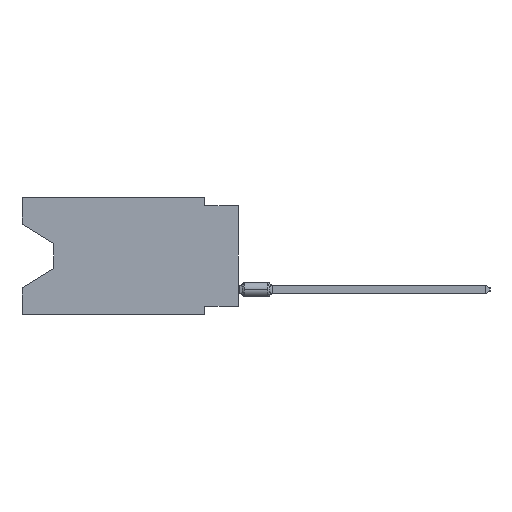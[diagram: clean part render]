
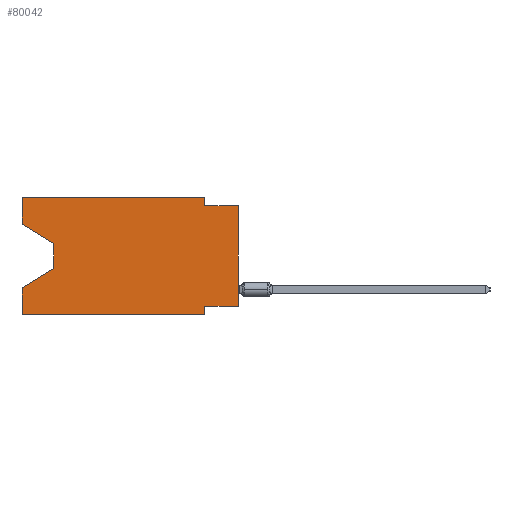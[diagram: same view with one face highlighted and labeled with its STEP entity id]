
A CAD part, left-side view. The second image highlights one B-rep face of the part: STEP entity #80042.
In plain terms, the highlighted planar face has unit normal (-1, 0, 0).
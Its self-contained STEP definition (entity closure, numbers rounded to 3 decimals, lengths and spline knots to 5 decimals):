
#1138 = CARTESIAN_POINT ( 'NONE',  ( 0., 0.645, 0. ) ) ;
#2386 = DIRECTION ( 'NONE',  ( 0., 0., -1. ) ) ;
#5109 = EDGE_CURVE ( 'NONE', #22256, #36637, #84031, .T. ) ;
#5518 = CARTESIAN_POINT ( 'NONE',  ( 0., 0.1, -0.35 ) ) ;
#6136 = VECTOR ( 'NONE', #38522, 39.37008 ) ;
#7480 = PLANE ( 'NONE',  #61533 ) ;
#9492 = VECTOR ( 'NONE', #92380, 39.37008 ) ;
#10822 = VERTEX_POINT ( 'NONE', #35926 ) ;
#14160 = CARTESIAN_POINT ( 'NONE',  ( 0., 0.645, 0. ) ) ;
#16501 = DIRECTION ( 'NONE',  ( 0., 0., 1. ) ) ;
#17333 = ORIENTED_EDGE ( 'NONE', *, *, #82261, .F. ) ;
#17602 = VECTOR ( 'NONE', #30311, 39.37008 ) ;
#21684 = ORIENTED_EDGE ( 'NONE', *, *, #89565, .F. ) ;
#22223 = CARTESIAN_POINT ( 'NONE',  ( 0., 0., -0.025 ) ) ;
#22256 = VERTEX_POINT ( 'NONE', #79996 ) ;
#23009 = DIRECTION ( 'NONE',  ( 0., -0.855, -0.519 ) ) ;
#23027 = EDGE_CURVE ( 'NONE', #95445, #22256, #58249, .T. ) ;
#23307 = DIRECTION ( 'NONE',  ( 1., 0., 0. ) ) ;
#24504 = ORIENTED_EDGE ( 'NONE', *, *, #60805, .T. ) ;
#24520 = CARTESIAN_POINT ( 'NONE',  ( 0., 0.645, -0.08025 ) ) ;
#25581 = LINE ( 'NONE', #94180, #74170 ) ;
#26067 = CARTESIAN_POINT ( 'NONE',  ( 0., 0.645, -0.26975 ) ) ;
#27872 = ORIENTED_EDGE ( 'NONE', *, *, #70523, .F. ) ;
#28115 = VERTEX_POINT ( 'NONE', #47231 ) ;
#30311 = DIRECTION ( 'NONE',  ( 0., 0., -1. ) ) ;
#30899 = EDGE_CURVE ( 'NONE', #37259, #60543, #55387, .T. ) ;
#31280 = DIRECTION ( 'NONE',  ( 0., 0.855, -0.519 ) ) ;
#31504 = EDGE_CURVE ( 'NONE', #95445, #28115, #61188, .T. ) ;
#31776 = LINE ( 'NONE', #55344, #57600 ) ;
#35926 = CARTESIAN_POINT ( 'NONE',  ( 0., 0.55, -0.212 ) ) ;
#36637 = VERTEX_POINT ( 'NONE', #5518 ) ;
#37259 = VERTEX_POINT ( 'NONE', #79303 ) ;
#38190 = FACE_OUTER_BOUND ( 'NONE', #45437, .T. ) ;
#38522 = DIRECTION ( 'NONE',  ( 0., -1., 0. ) ) ;
#39953 = CARTESIAN_POINT ( 'NONE',  ( 0., 0.1, -0.025 ) ) ;
#40557 = VECTOR ( 'NONE', #89088, 39.37008 ) ;
#43129 = DIRECTION ( 'NONE',  ( 0., -1., 0. ) ) ;
#43143 = ORIENTED_EDGE ( 'NONE', *, *, #5109, .F. ) ;
#45437 = EDGE_LOOP ( 'NONE', ( #86370, #55375, #54980, #17333, #24504, #43143, #93925, #67899, #27872, #21684, #79628, #53374 ) ) ;
#46561 = EDGE_CURVE ( 'NONE', #88113, #84845, #84922, .T. ) ;
#47231 = CARTESIAN_POINT ( 'NONE',  ( 0., 0., -0.025 ) ) ;
#47615 = DIRECTION ( 'NONE',  ( 0., 0., -1. ) ) ;
#49621 = EDGE_CURVE ( 'NONE', #88113, #37259, #63076, .T. ) ;
#50773 = EDGE_CURVE ( 'NONE', #84845, #10822, #65829, .T. ) ;
#51601 = CARTESIAN_POINT ( 'NONE',  ( 0., 0., -0.325 ) ) ;
#51664 = CARTESIAN_POINT ( 'NONE',  ( 0., 0.645, -0.08025 ) ) ;
#53374 = ORIENTED_EDGE ( 'NONE', *, *, #49621, .F. ) ;
#53877 = VECTOR ( 'NONE', #43129, 39.37008 ) ;
#54980 = ORIENTED_EDGE ( 'NONE', *, *, #63951, .T. ) ;
#55344 = CARTESIAN_POINT ( 'NONE',  ( 0., 0.55, -0.212 ) ) ;
#55375 = ORIENTED_EDGE ( 'NONE', *, *, #50773, .T. ) ;
#55387 = LINE ( 'NONE', #1138, #6136 ) ;
#55412 = CARTESIAN_POINT ( 'NONE',  ( 0., 0.645, 0. ) ) ;
#55565 = VECTOR ( 'NONE', #68803, 39.37008 ) ;
#57600 = VECTOR ( 'NONE', #31280, 39.37008 ) ;
#58249 = LINE ( 'NONE', #51601, #89043 ) ;
#58957 = VECTOR ( 'NONE', #2386, 39.37008 ) ;
#60019 = CARTESIAN_POINT ( 'NONE',  ( 0., 0.645, -0.35 ) ) ;
#60088 = CARTESIAN_POINT ( 'NONE',  ( 0., 0., -0.325 ) ) ;
#60543 = VERTEX_POINT ( 'NONE', #77472 ) ;
#60805 = EDGE_CURVE ( 'NONE', #68215, #36637, #90189, .T. ) ;
#61188 = LINE ( 'NONE', #101075, #9492 ) ;
#61533 = AXIS2_PLACEMENT_3D ( 'NONE', #14160, #23307, #85231 ) ;
#63076 = LINE ( 'NONE', #55412, #76707 ) ;
#63951 = EDGE_CURVE ( 'NONE', #10822, #79294, #31776, .T. ) ;
#65829 = LINE ( 'NONE', #72479, #58957 ) ;
#66440 = DIRECTION ( 'NONE',  ( 0., 1., 0. ) ) ;
#67705 = CARTESIAN_POINT ( 'NONE',  ( 0., 0.1, -0.35 ) ) ;
#67899 = ORIENTED_EDGE ( 'NONE', *, *, #31504, .T. ) ;
#68215 = VERTEX_POINT ( 'NONE', #100474 ) ;
#68803 = DIRECTION ( 'NONE',  ( 0., -1., 0. ) ) ;
#70523 = EDGE_CURVE ( 'NONE', #73658, #28115, #83628, .T. ) ;
#72479 = CARTESIAN_POINT ( 'NONE',  ( 0., 0.55, -0.138 ) ) ;
#73658 = VERTEX_POINT ( 'NONE', #39953 ) ;
#74170 = VECTOR ( 'NONE', #47615, 39.37008 ) ;
#74785 = CARTESIAN_POINT ( 'NONE',  ( 0., 0.645, 0. ) ) ;
#76707 = VECTOR ( 'NONE', #16501, 39.37008 ) ;
#77472 = CARTESIAN_POINT ( 'NONE',  ( 0., 0.1, 0. ) ) ;
#79294 = VERTEX_POINT ( 'NONE', #26067 ) ;
#79303 = CARTESIAN_POINT ( 'NONE',  ( 0., 0.645, 0. ) ) ;
#79628 = ORIENTED_EDGE ( 'NONE', *, *, #30899, .F. ) ;
#79996 = CARTESIAN_POINT ( 'NONE',  ( 0., 0.1, -0.325 ) ) ;
#80042 = ADVANCED_FACE ( 'NONE', ( #38190 ), #7480, .F. ) ;
#82261 = EDGE_CURVE ( 'NONE', #68215, #79294, #98779, .T. ) ;
#83628 = LINE ( 'NONE', #22223, #55565 ) ;
#84031 = LINE ( 'NONE', #67705, #17602 ) ;
#84845 = VERTEX_POINT ( 'NONE', #92891 ) ;
#84922 = LINE ( 'NONE', #24520, #99134 ) ;
#85231 = DIRECTION ( 'NONE',  ( 0., 0., -1. ) ) ;
#86370 = ORIENTED_EDGE ( 'NONE', *, *, #46561, .T. ) ;
#88113 = VERTEX_POINT ( 'NONE', #51664 ) ;
#89043 = VECTOR ( 'NONE', #66440, 39.37008 ) ;
#89088 = DIRECTION ( 'NONE',  ( 0., 0., 1. ) ) ;
#89565 = EDGE_CURVE ( 'NONE', #60543, #73658, #25581, .T. ) ;
#90189 = LINE ( 'NONE', #60019, #53877 ) ;
#92380 = DIRECTION ( 'NONE',  ( 0., 0., 1. ) ) ;
#92891 = CARTESIAN_POINT ( 'NONE',  ( 0., 0.55, -0.138 ) ) ;
#93925 = ORIENTED_EDGE ( 'NONE', *, *, #23027, .F. ) ;
#94180 = CARTESIAN_POINT ( 'NONE',  ( 0., 0.1, 0. ) ) ;
#95445 = VERTEX_POINT ( 'NONE', #60088 ) ;
#98779 = LINE ( 'NONE', #74785, #40557 ) ;
#99134 = VECTOR ( 'NONE', #23009, 39.37008 ) ;
#100474 = CARTESIAN_POINT ( 'NONE',  ( 0., 0.645, -0.35 ) ) ;
#101075 = CARTESIAN_POINT ( 'NONE',  ( 0., 0., 0. ) ) ;
